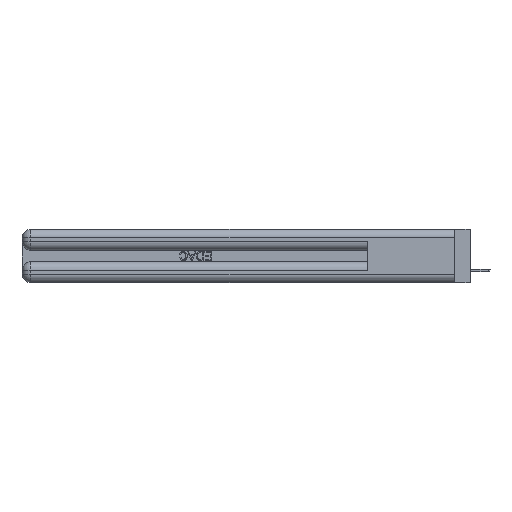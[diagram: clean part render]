
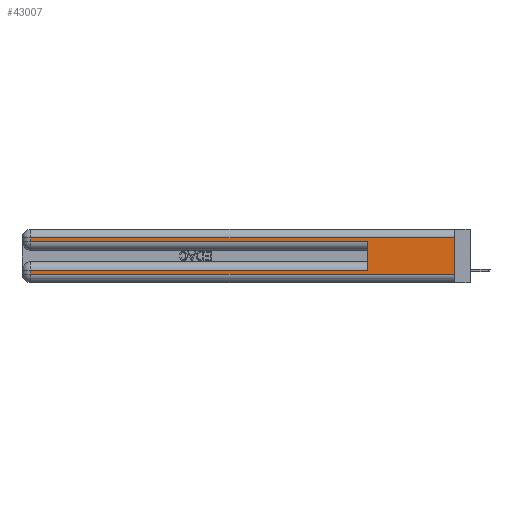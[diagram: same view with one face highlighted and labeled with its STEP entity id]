
A CAD part, left-side view. The second image highlights one B-rep face of the part: STEP entity #43007.
In plain terms, the highlighted planar face has unit normal (-1, 0, 0).
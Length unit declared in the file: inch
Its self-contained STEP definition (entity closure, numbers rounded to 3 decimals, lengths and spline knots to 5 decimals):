
#2508 = DIRECTION ( 'NONE',  ( 0., -1., 0. ) ) ;
#3373 = DIRECTION ( 'NONE',  ( 0., 0., 1. ) ) ;
#4898 = CARTESIAN_POINT ( 'NONE',  ( 0., 0., 0.06 ) ) ;
#5144 = EDGE_CURVE ( 'NONE', #5860, #14483, #25299, .T. ) ;
#5860 = VERTEX_POINT ( 'NONE', #47502 ) ;
#6092 = ORIENTED_EDGE ( 'NONE', *, *, #27945, .T. ) ;
#7023 = VERTEX_POINT ( 'NONE', #22835 ) ;
#9386 = DIRECTION ( 'NONE',  ( 1., 0., 0. ) ) ;
#10362 = LINE ( 'NONE', #14918, #37980 ) ;
#10813 = DIRECTION ( 'NONE',  ( 0., 0., -1. ) ) ;
#12897 = AXIS2_PLACEMENT_3D ( 'NONE', #18213, #9386, #13933 ) ;
#13372 = EDGE_CURVE ( 'NONE', #16399, #49034, #17559, .T. ) ;
#13783 = VERTEX_POINT ( 'NONE', #41694 ) ;
#13933 = DIRECTION ( 'NONE',  ( 0., 0., -1. ) ) ;
#14483 = VERTEX_POINT ( 'NONE', #19536 ) ;
#14918 = CARTESIAN_POINT ( 'NONE',  ( 0., 0., 0.085 ) ) ;
#15973 = LINE ( 'NONE', #16501, #32765 ) ;
#16399 = VERTEX_POINT ( 'NONE', #25211 ) ;
#16501 = CARTESIAN_POINT ( 'NONE',  ( 0., 0.6, 0.145 ) ) ;
#16665 = ORIENTED_EDGE ( 'NONE', *, *, #5144, .T. ) ;
#17559 = LINE ( 'NONE', #29896, #23987 ) ;
#18213 = CARTESIAN_POINT ( 'NONE',  ( 0., 0., 0.37 ) ) ;
#18631 = EDGE_CURVE ( 'NONE', #7023, #5860, #19656, .T. ) ;
#18745 = ORIENTED_EDGE ( 'NONE', *, *, #13372, .T. ) ;
#19258 = VECTOR ( 'NONE', #24121, 39.37008 ) ;
#19536 = CARTESIAN_POINT ( 'NONE',  ( 0., 0., 0.06 ) ) ;
#19656 = LINE ( 'NONE', #23434, #52229 ) ;
#19822 = CARTESIAN_POINT ( 'NONE',  ( 0., 0., 0.37 ) ) ;
#22003 = PLANE ( 'NONE',  #12897 ) ;
#22600 = CARTESIAN_POINT ( 'NONE',  ( 0., 0.6, 0.285 ) ) ;
#22835 = CARTESIAN_POINT ( 'NONE',  ( 0., 2.94, 0.085 ) ) ;
#23434 = CARTESIAN_POINT ( 'NONE',  ( 0., 2.94, 0.37 ) ) ;
#23987 = VECTOR ( 'NONE', #46324, 39.37008 ) ;
#24107 = EDGE_CURVE ( 'NONE', #45796, #7023, #10362, .T. ) ;
#24121 = DIRECTION ( 'NONE',  ( 0., 0., -1. ) ) ;
#24152 = EDGE_CURVE ( 'NONE', #45796, #39115, #15973, .T. ) ;
#25090 = CARTESIAN_POINT ( 'NONE',  ( 0., 2.94, 0.31 ) ) ;
#25211 = CARTESIAN_POINT ( 'NONE',  ( 0., 0., 0.31 ) ) ;
#25291 = ORIENTED_EDGE ( 'NONE', *, *, #24107, .T. ) ;
#25299 = LINE ( 'NONE', #4898, #42003 ) ;
#26222 = CARTESIAN_POINT ( 'NONE',  ( 0., 0.6, 0.085 ) ) ;
#26270 = EDGE_LOOP ( 'NONE', ( #50287, #18745, #44678, #6092, #52724, #25291, #37926, #16665 ) ) ;
#26728 = DIRECTION ( 'NONE',  ( 0., 1., 0. ) ) ;
#27453 = DIRECTION ( 'NONE',  ( 0., 0., -1. ) ) ;
#27848 = VECTOR ( 'NONE', #10813, 39.37008 ) ;
#27945 = EDGE_CURVE ( 'NONE', #13783, #39115, #39333, .T. ) ;
#29496 = FACE_OUTER_BOUND ( 'NONE', #26270, .T. ) ;
#29896 = CARTESIAN_POINT ( 'NONE',  ( 0., 0., 0.31 ) ) ;
#32765 = VECTOR ( 'NONE', #3373, 39.37008 ) ;
#34316 = EDGE_CURVE ( 'NONE', #16399, #14483, #48300, .T. ) ;
#34736 = LINE ( 'NONE', #35526, #27848 ) ;
#35526 = CARTESIAN_POINT ( 'NONE',  ( 0., 2.94, 0.37 ) ) ;
#36072 = CARTESIAN_POINT ( 'NONE',  ( 0., 0., 0.285 ) ) ;
#37926 = ORIENTED_EDGE ( 'NONE', *, *, #18631, .T. ) ;
#37980 = VECTOR ( 'NONE', #26728, 39.37008 ) ;
#38242 = VECTOR ( 'NONE', #2508, 39.37008 ) ;
#39115 = VERTEX_POINT ( 'NONE', #22600 ) ;
#39333 = LINE ( 'NONE', #36072, #38242 ) ;
#41694 = CARTESIAN_POINT ( 'NONE',  ( 0., 2.94, 0.285 ) ) ;
#42003 = VECTOR ( 'NONE', #45994, 39.37008 ) ;
#43007 = ADVANCED_FACE ( 'NONE', ( #29496 ), #22003, .F. ) ;
#44678 = ORIENTED_EDGE ( 'NONE', *, *, #50433, .T. ) ;
#45796 = VERTEX_POINT ( 'NONE', #26222 ) ;
#45994 = DIRECTION ( 'NONE',  ( 0., -1., 0. ) ) ;
#46324 = DIRECTION ( 'NONE',  ( 0., 1., 0. ) ) ;
#47502 = CARTESIAN_POINT ( 'NONE',  ( 0., 2.94, 0.06 ) ) ;
#48300 = LINE ( 'NONE', #19822, #19258 ) ;
#49034 = VERTEX_POINT ( 'NONE', #25090 ) ;
#50287 = ORIENTED_EDGE ( 'NONE', *, *, #34316, .F. ) ;
#50433 = EDGE_CURVE ( 'NONE', #49034, #13783, #34736, .T. ) ;
#52229 = VECTOR ( 'NONE', #27453, 39.37008 ) ;
#52724 = ORIENTED_EDGE ( 'NONE', *, *, #24152, .F. ) ;
